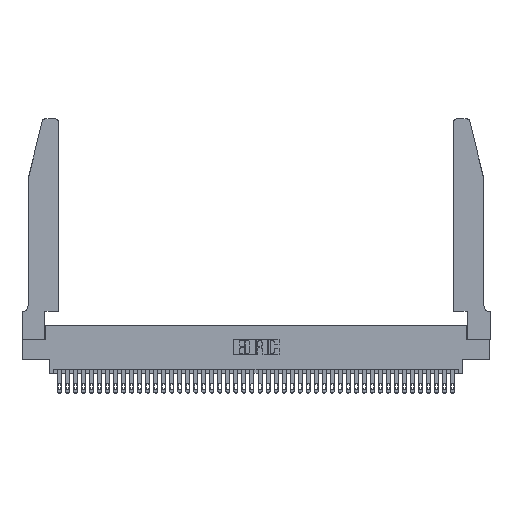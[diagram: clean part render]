
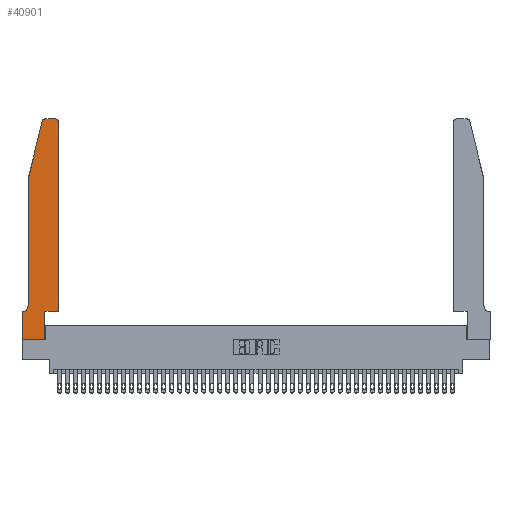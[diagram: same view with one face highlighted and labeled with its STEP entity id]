
A CAD part, top view. The second image highlights one B-rep face of the part: STEP entity #40901.
In plain terms, the highlighted planar face has unit normal (0, 0, 1).
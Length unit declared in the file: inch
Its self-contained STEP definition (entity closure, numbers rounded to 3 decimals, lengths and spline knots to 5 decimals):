
#810 = CARTESIAN_POINT ( 'NONE',  ( 0.4505, 0.35, 0.37 ) ) ;
#1446 = DIRECTION ( 'NONE',  ( 1., 0., 0. ) ) ;
#1647 = VERTEX_POINT ( 'NONE', #2904 ) ;
#1826 = VERTEX_POINT ( 'NONE', #30943 ) ;
#1843 = DIRECTION ( 'NONE',  ( 0., 1., 0. ) ) ;
#2186 = ORIENTED_EDGE ( 'NONE', *, *, #36158, .T. ) ;
#2276 = CARTESIAN_POINT ( 'NONE',  ( 0., 0.35, 0.37 ) ) ;
#2410 = DIRECTION ( 'NONE',  ( 0., -1., 0. ) ) ;
#2631 = ORIENTED_EDGE ( 'NONE', *, *, #21557, .T. ) ;
#2904 = CARTESIAN_POINT ( 'NONE',  ( 0.25487, 2.72718, 0.37 ) ) ;
#3312 = DIRECTION ( 'NONE',  ( 0., 0., 1. ) ) ;
#3593 = DIRECTION ( 'NONE',  ( 1., 0., 0. ) ) ;
#3772 = LINE ( 'NONE', #30443, #38620 ) ;
#4402 = AXIS2_PLACEMENT_3D ( 'NONE', #32974, #42845, #16164 ) ;
#5499 = EDGE_CURVE ( 'NONE', #1647, #11574, #17818, .T. ) ;
#5757 = VERTEX_POINT ( 'NONE', #24238 ) ;
#5794 = CARTESIAN_POINT ( 'NONE',  ( 0., 0., 0.37 ) ) ;
#6334 = VECTOR ( 'NONE', #16094, 39.37008 ) ;
#7552 = VECTOR ( 'NONE', #1843, 39.37008 ) ;
#8372 = ORIENTED_EDGE ( 'NONE', *, *, #20632, .T. ) ;
#8504 = DIRECTION ( 'NONE',  ( -0.239, -0.971, 0. ) ) ;
#8582 = VERTEX_POINT ( 'NONE', #32819 ) ;
#9308 = CARTESIAN_POINT ( 'NONE',  ( 0.0755, 2., 0.37 ) ) ;
#9435 = PLANE ( 'NONE',  #22621 ) ;
#10825 = DIRECTION ( 'NONE',  ( 0., -1., 0. ) ) ;
#11343 = CARTESIAN_POINT ( 'NONE',  ( 0.0755, 0.42, 0.37 ) ) ;
#11574 = VERTEX_POINT ( 'NONE', #9308 ) ;
#11882 = DIRECTION ( 'NONE',  ( 0., 0., 1. ) ) ;
#12299 = ORIENTED_EDGE ( 'NONE', *, *, #29873, .T. ) ;
#12874 = DIRECTION ( 'NONE',  ( -1., 0., 0. ) ) ;
#13040 = VECTOR ( 'NONE', #23802, 39.37008 ) ;
#13047 = CARTESIAN_POINT ( 'NONE',  ( 0., 0., 0.37 ) ) ;
#13318 = LINE ( 'NONE', #38293, #7552 ) ;
#13793 = ORIENTED_EDGE ( 'NONE', *, *, #17612, .T. ) ;
#13902 = VECTOR ( 'NONE', #10825, 39.37008 ) ;
#14941 = AXIS2_PLACEMENT_3D ( 'NONE', #31742, #11882, #39604 ) ;
#15197 = LINE ( 'NONE', #22618, #6334 ) ;
#15319 = EDGE_LOOP ( 'NONE', ( #13793, #2631, #37609, #2186, #36389, #30296, #42722, #12299, #35582, #8372, #31284, #28100 ) ) ;
#16094 = DIRECTION ( 'NONE',  ( 1., 0., 0. ) ) ;
#16164 = DIRECTION ( 'NONE',  ( -1., 0., 0. ) ) ;
#17030 = VECTOR ( 'NONE', #40876, 39.37008 ) ;
#17351 = CARTESIAN_POINT ( 'NONE',  ( 0.0755, 0.35, 0.37 ) ) ;
#17612 = EDGE_CURVE ( 'NONE', #20844, #5757, #33766, .T. ) ;
#17818 = LINE ( 'NONE', #31594, #29810 ) ;
#18976 = VERTEX_POINT ( 'NONE', #2276 ) ;
#19534 = CARTESIAN_POINT ( 'NONE',  ( 0.2865, 0., 0.37 ) ) ;
#20186 = VERTEX_POINT ( 'NONE', #810 ) ;
#20616 = LINE ( 'NONE', #13047, #13902 ) ;
#20632 = EDGE_CURVE ( 'NONE', #8582, #20186, #3772, .T. ) ;
#20844 = VERTEX_POINT ( 'NONE', #24484 ) ;
#20913 = CIRCLE ( 'NONE', #30370, 0.03 ) ;
#21521 = DIRECTION ( 'NONE',  ( 0., 0., 1. ) ) ;
#21557 = EDGE_CURVE ( 'NONE', #5757, #1647, #34891, .T. ) ;
#21766 = VERTEX_POINT ( 'NONE', #21786 ) ;
#21786 = CARTESIAN_POINT ( 'NONE',  ( 0.4505, 2.72, 0.37 ) ) ;
#22618 = CARTESIAN_POINT ( 'NONE',  ( 0., 0., 0.37 ) ) ;
#22621 = AXIS2_PLACEMENT_3D ( 'NONE', #39159, #3312, #36358 ) ;
#23290 = EDGE_CURVE ( 'NONE', #24475, #8582, #37901, .T. ) ;
#23802 = DIRECTION ( 'NONE',  ( 0., 1., 0. ) ) ;
#24238 = CARTESIAN_POINT ( 'NONE',  ( 0.284, 2.75, 0.37 ) ) ;
#24475 = VERTEX_POINT ( 'NONE', #19534 ) ;
#24484 = CARTESIAN_POINT ( 'NONE',  ( 0.4205, 2.75, 0.37 ) ) ;
#24640 = EDGE_CURVE ( 'NONE', #18976, #40754, #20616, .T. ) ;
#25228 = LINE ( 'NONE', #29434, #36087 ) ;
#25699 = CIRCLE ( 'NONE', #4402, 0.07 ) ;
#26198 = EDGE_CURVE ( 'NONE', #1826, #18976, #38354, .T. ) ;
#27875 = EDGE_CURVE ( 'NONE', #20186, #21766, #13318, .T. ) ;
#28100 = ORIENTED_EDGE ( 'NONE', *, *, #40171, .T. ) ;
#29434 = CARTESIAN_POINT ( 'NONE',  ( 0.0755, 2., 0.37 ) ) ;
#29617 = VECTOR ( 'NONE', #12874, 39.37008 ) ;
#29683 = VERTEX_POINT ( 'NONE', #11343 ) ;
#29810 = VECTOR ( 'NONE', #8504, 39.37008 ) ;
#29873 = EDGE_CURVE ( 'NONE', #40754, #24475, #15197, .T. ) ;
#30296 = ORIENTED_EDGE ( 'NONE', *, *, #26198, .T. ) ;
#30370 = AXIS2_PLACEMENT_3D ( 'NONE', #34416, #21521, #1446 ) ;
#30443 = CARTESIAN_POINT ( 'NONE',  ( 0.4505, 0.35, 0.37 ) ) ;
#30943 = CARTESIAN_POINT ( 'NONE',  ( 0.0055, 0.35, 0.37 ) ) ;
#31284 = ORIENTED_EDGE ( 'NONE', *, *, #27875, .T. ) ;
#31594 = CARTESIAN_POINT ( 'NONE',  ( 0.0755, 2., 0.37 ) ) ;
#31742 = CARTESIAN_POINT ( 'NONE',  ( 0.284, 2.72, 0.37 ) ) ;
#32720 = CARTESIAN_POINT ( 'NONE',  ( 0.2605, 2.75, 0.37 ) ) ;
#32819 = CARTESIAN_POINT ( 'NONE',  ( 0.2865, 0.35, 0.37 ) ) ;
#32974 = CARTESIAN_POINT ( 'NONE',  ( 0.0055, 0.42, 0.37 ) ) ;
#33766 = LINE ( 'NONE', #32720, #29617 ) ;
#34396 = CARTESIAN_POINT ( 'NONE',  ( 0.2865, 0.35, 0.37 ) ) ;
#34416 = CARTESIAN_POINT ( 'NONE',  ( 0.4205, 2.72, 0.37 ) ) ;
#34891 = CIRCLE ( 'NONE', #14941, 0.03 ) ;
#35582 = ORIENTED_EDGE ( 'NONE', *, *, #23290, .T. ) ;
#36087 = VECTOR ( 'NONE', #2410, 39.37008 ) ;
#36158 = EDGE_CURVE ( 'NONE', #11574, #29683, #25228, .T. ) ;
#36358 = DIRECTION ( 'NONE',  ( 1., 0., 0. ) ) ;
#36389 = ORIENTED_EDGE ( 'NONE', *, *, #36798, .T. ) ;
#36798 = EDGE_CURVE ( 'NONE', #29683, #1826, #25699, .T. ) ;
#37609 = ORIENTED_EDGE ( 'NONE', *, *, #5499, .T. ) ;
#37901 = LINE ( 'NONE', #34396, #13040 ) ;
#38293 = CARTESIAN_POINT ( 'NONE',  ( 0.4505, 0.35, 0.37 ) ) ;
#38354 = LINE ( 'NONE', #17351, #17030 ) ;
#38620 = VECTOR ( 'NONE', #3593, 39.37008 ) ;
#39159 = CARTESIAN_POINT ( 'NONE',  ( 0., 0.35, 0.37 ) ) ;
#39604 = DIRECTION ( 'NONE',  ( 1., 0., 0. ) ) ;
#40171 = EDGE_CURVE ( 'NONE', #21766, #20844, #20913, .T. ) ;
#40754 = VERTEX_POINT ( 'NONE', #5794 ) ;
#40876 = DIRECTION ( 'NONE',  ( -1., 0., 0. ) ) ;
#40901 = ADVANCED_FACE ( 'NONE', ( #42132 ), #9435, .T. ) ;
#42132 = FACE_OUTER_BOUND ( 'NONE', #15319, .T. ) ;
#42722 = ORIENTED_EDGE ( 'NONE', *, *, #24640, .T. ) ;
#42845 = DIRECTION ( 'NONE',  ( 0., 0., -1. ) ) ;
